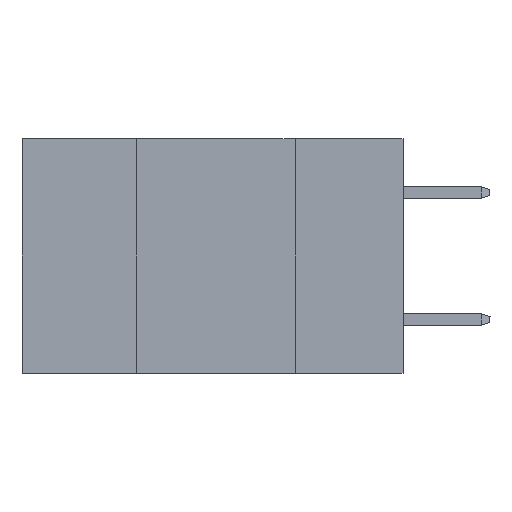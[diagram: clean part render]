
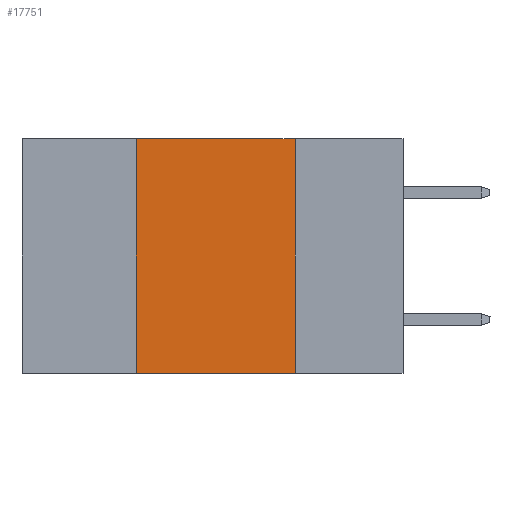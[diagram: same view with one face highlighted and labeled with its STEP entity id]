
A CAD part, left-side view. The second image highlights one B-rep face of the part: STEP entity #17751.
In plain terms, the highlighted planar face has unit normal (-1, 0, 0).
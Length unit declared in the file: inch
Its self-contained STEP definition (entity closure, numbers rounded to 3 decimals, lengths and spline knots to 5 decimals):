
#693 = VERTEX_POINT ( 'NONE', #29829 ) ;
#1273 = DIRECTION ( 'NONE',  ( 0., 0., 1. ) ) ;
#2020 = ORIENTED_EDGE ( 'NONE', *, *, #19753, .T. ) ;
#4101 = CARTESIAN_POINT ( 'NONE',  ( 0., 0.17, -0.37 ) ) ;
#4117 = VERTEX_POINT ( 'NONE', #18575 ) ;
#4402 = EDGE_CURVE ( 'NONE', #4117, #693, #22022, .T. ) ;
#5732 = VECTOR ( 'NONE', #1273, 39.37008 ) ;
#5842 = DIRECTION ( 'NONE',  ( 0., 0., -1. ) ) ;
#5858 = DIRECTION ( 'NONE',  ( 0., -1., 0. ) ) ;
#6429 = LINE ( 'NONE', #17942, #15945 ) ;
#8082 = VERTEX_POINT ( 'NONE', #26574 ) ;
#8113 = CARTESIAN_POINT ( 'NONE',  ( 0., 0.6, -0.37 ) ) ;
#8201 = EDGE_CURVE ( 'NONE', #8082, #23433, #6429, .T. ) ;
#8685 = CARTESIAN_POINT ( 'NONE',  ( 0., 0.6, 0. ) ) ;
#8967 = ORIENTED_EDGE ( 'NONE', *, *, #4402, .F. ) ;
#9387 = EDGE_LOOP ( 'NONE', ( #16559, #13116, #8967, #2020 ) ) ;
#10380 = DIRECTION ( 'NONE',  ( 1., 0., 0. ) ) ;
#10837 = EDGE_CURVE ( 'NONE', #693, #8082, #27183, .T. ) ;
#11429 = DIRECTION ( 'NONE',  ( 0., -1., 0. ) ) ;
#12957 = CARTESIAN_POINT ( 'NONE',  ( 0., 0.6, 0. ) ) ;
#13116 = ORIENTED_EDGE ( 'NONE', *, *, #10837, .F. ) ;
#13835 = DIRECTION ( 'NONE',  ( 0., 0., -1. ) ) ;
#15945 = VECTOR ( 'NONE', #13835, 39.37008 ) ;
#16559 = ORIENTED_EDGE ( 'NONE', *, *, #8201, .F. ) ;
#17751 = ADVANCED_FACE ( 'NONE', ( #22171 ), #26583, .F. ) ;
#17942 = CARTESIAN_POINT ( 'NONE',  ( 0., 0.17, 0. ) ) ;
#18575 = CARTESIAN_POINT ( 'NONE',  ( 0., 0.42, -0.37 ) ) ;
#19753 = EDGE_CURVE ( 'NONE', #4117, #23433, #26597, .T. ) ;
#20312 = VECTOR ( 'NONE', #11429, 39.37008 ) ;
#20700 = VECTOR ( 'NONE', #5858, 39.37008 ) ;
#22022 = LINE ( 'NONE', #26742, #5732 ) ;
#22171 = FACE_OUTER_BOUND ( 'NONE', #9387, .T. ) ;
#23433 = VERTEX_POINT ( 'NONE', #4101 ) ;
#26574 = CARTESIAN_POINT ( 'NONE',  ( 0., 0.17, 0. ) ) ;
#26583 = PLANE ( 'NONE',  #28270 ) ;
#26597 = LINE ( 'NONE', #8113, #20700 ) ;
#26742 = CARTESIAN_POINT ( 'NONE',  ( 0., 0.42, 0. ) ) ;
#27183 = LINE ( 'NONE', #8685, #20312 ) ;
#28270 = AXIS2_PLACEMENT_3D ( 'NONE', #12957, #10380, #5842 ) ;
#29829 = CARTESIAN_POINT ( 'NONE',  ( 0., 0.42, 0. ) ) ;
